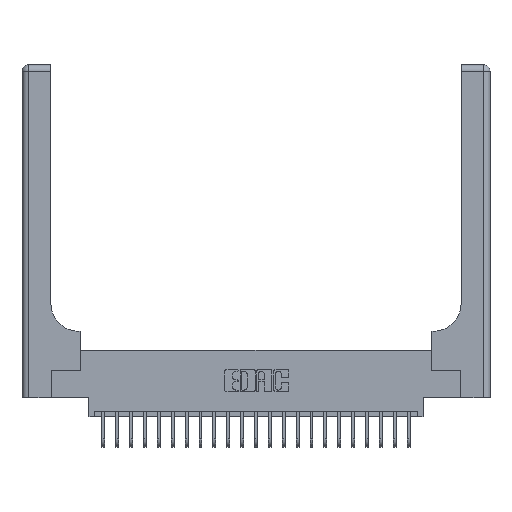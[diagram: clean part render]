
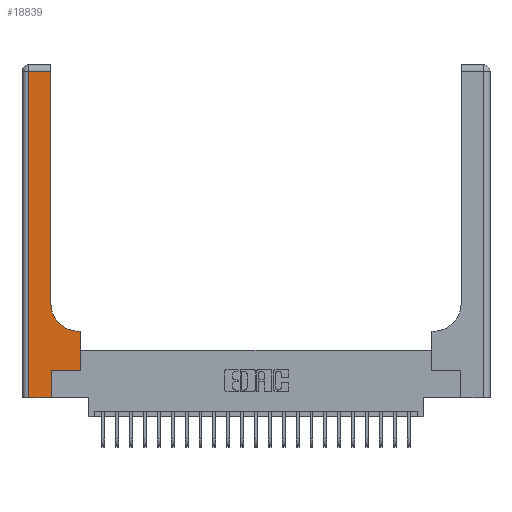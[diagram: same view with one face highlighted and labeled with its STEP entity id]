
A CAD part, top view. The second image highlights one B-rep face of the part: STEP entity #18839.
In plain terms, the highlighted planar face has unit normal (0, 0, 1).
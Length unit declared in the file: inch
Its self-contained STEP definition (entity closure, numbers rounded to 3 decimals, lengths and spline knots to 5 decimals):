
#45 = CARTESIAN_POINT ( 'NONE',  ( 0.51, 0.85, 0.37 ) ) ;
#279 = VERTEX_POINT ( 'NONE', #16182 ) ;
#375 = EDGE_CURVE ( 'NONE', #14481, #13839, #10200, .T. ) ;
#930 = LINE ( 'NONE', #8889, #1818 ) ;
#1572 = EDGE_CURVE ( 'NONE', #6969, #279, #13695, .T. ) ;
#1818 = VECTOR ( 'NONE', #12996, 39.37008 ) ;
#1852 = CARTESIAN_POINT ( 'NONE',  ( 0.06, 2.94, 0.37 ) ) ;
#2109 = ORIENTED_EDGE ( 'NONE', *, *, #14729, .T. ) ;
#2408 = DIRECTION ( 'NONE',  ( 1., 0., 0. ) ) ;
#2704 = VECTOR ( 'NONE', #4896, 39.37008 ) ;
#2709 = VERTEX_POINT ( 'NONE', #18155 ) ;
#3014 = CARTESIAN_POINT ( 'NONE',  ( 0.265, 0., 0.37 ) ) ;
#3131 = LINE ( 'NONE', #18366, #6955 ) ;
#3745 = EDGE_CURVE ( 'NONE', #18095, #14481, #22326, .T. ) ;
#4564 = ORIENTED_EDGE ( 'NONE', *, *, #11835, .T. ) ;
#4658 = LINE ( 'NONE', #8134, #10041 ) ;
#4896 = DIRECTION ( 'NONE',  ( 0., 1., 0. ) ) ;
#5174 = CARTESIAN_POINT ( 'NONE',  ( 0.26, 0.6, 0.37 ) ) ;
#5315 = AXIS2_PLACEMENT_3D ( 'NONE', #45, #13384, #21041 ) ;
#5909 = DIRECTION ( 'NONE',  ( 0., 0., -1. ) ) ;
#6440 = CARTESIAN_POINT ( 'NONE',  ( 0.528, 0.25, 0.37 ) ) ;
#6832 = DIRECTION ( 'NONE',  ( 1., 0., 0. ) ) ;
#6955 = VECTOR ( 'NONE', #16441, 39.37008 ) ;
#6969 = VERTEX_POINT ( 'NONE', #14373 ) ;
#7077 = DIRECTION ( 'NONE',  ( 0., 1., 0. ) ) ;
#7205 = VERTEX_POINT ( 'NONE', #1852 ) ;
#7296 = ORIENTED_EDGE ( 'NONE', *, *, #14107, .T. ) ;
#8134 = CARTESIAN_POINT ( 'NONE',  ( 0.265, 0.25, 0.37 ) ) ;
#8305 = ORIENTED_EDGE ( 'NONE', *, *, #375, .T. ) ;
#8889 = CARTESIAN_POINT ( 'NONE',  ( 0., 2.94, 0.37 ) ) ;
#9319 = EDGE_LOOP ( 'NONE', ( #18360, #21940, #4564, #7296, #2109, #10422, #13967, #8305, #23266 ) ) ;
#9759 = DIRECTION ( 'NONE',  ( -1., 0., 0. ) ) ;
#10041 = VECTOR ( 'NONE', #2408, 39.37008 ) ;
#10200 = LINE ( 'NONE', #5174, #20629 ) ;
#10422 = ORIENTED_EDGE ( 'NONE', *, *, #22167, .T. ) ;
#10571 = CARTESIAN_POINT ( 'NONE',  ( 0.06, 0., 0.37 ) ) ;
#10867 = EDGE_CURVE ( 'NONE', #13839, #6969, #19542, .T. ) ;
#11835 = EDGE_CURVE ( 'NONE', #7205, #21996, #3131, .T. ) ;
#11915 = VECTOR ( 'NONE', #7077, 39.37008 ) ;
#11971 = DIRECTION ( 'NONE',  ( 0., 1., 0. ) ) ;
#12144 = VECTOR ( 'NONE', #11971, 39.37008 ) ;
#12259 = VECTOR ( 'NONE', #6832, 39.37008 ) ;
#12650 = CARTESIAN_POINT ( 'NONE',  ( 0.528, 0.25, 0.37 ) ) ;
#12725 = CARTESIAN_POINT ( 'NONE',  ( 0.51, 0.6, 0.37 ) ) ;
#12996 = DIRECTION ( 'NONE',  ( -1., 0., 0. ) ) ;
#13286 = CARTESIAN_POINT ( 'NONE',  ( 0.265, 0., 0.37 ) ) ;
#13384 = DIRECTION ( 'NONE',  ( 0., 0., -1. ) ) ;
#13695 = LINE ( 'NONE', #22455, #11915 ) ;
#13818 = EDGE_CURVE ( 'NONE', #279, #7205, #930, .T. ) ;
#13839 = VERTEX_POINT ( 'NONE', #12725 ) ;
#13967 = ORIENTED_EDGE ( 'NONE', *, *, #3745, .T. ) ;
#14107 = EDGE_CURVE ( 'NONE', #21996, #15468, #17940, .T. ) ;
#14373 = CARTESIAN_POINT ( 'NONE',  ( 0.26, 0.85, 0.37 ) ) ;
#14481 = VERTEX_POINT ( 'NONE', #17111 ) ;
#14729 = EDGE_CURVE ( 'NONE', #15468, #2709, #14930, .T. ) ;
#14930 = LINE ( 'NONE', #3014, #2704 ) ;
#15468 = VERTEX_POINT ( 'NONE', #13286 ) ;
#15819 = FACE_OUTER_BOUND ( 'NONE', #9319, .T. ) ;
#16182 = CARTESIAN_POINT ( 'NONE',  ( 0.26, 2.94, 0.37 ) ) ;
#16441 = DIRECTION ( 'NONE',  ( 0., -1., 0. ) ) ;
#17111 = CARTESIAN_POINT ( 'NONE',  ( 0.528, 0.6, 0.37 ) ) ;
#17300 = PLANE ( 'NONE',  #23432 ) ;
#17380 = CARTESIAN_POINT ( 'NONE',  ( 0., 3., 0.37 ) ) ;
#17940 = LINE ( 'NONE', #23045, #12259 ) ;
#18095 = VERTEX_POINT ( 'NONE', #12650 ) ;
#18155 = CARTESIAN_POINT ( 'NONE',  ( 0.265, 0.25, 0.37 ) ) ;
#18360 = ORIENTED_EDGE ( 'NONE', *, *, #1572, .T. ) ;
#18366 = CARTESIAN_POINT ( 'NONE',  ( 0.06, 3., 0.37 ) ) ;
#18497 = DIRECTION ( 'NONE',  ( -1., 0., 0. ) ) ;
#18839 = ADVANCED_FACE ( 'NONE', ( #15819 ), #17300, .F. ) ;
#19542 = CIRCLE ( 'NONE', #5315, 0.25 ) ;
#20629 = VECTOR ( 'NONE', #18497, 39.37008 ) ;
#21041 = DIRECTION ( 'NONE',  ( 1., 0., 0. ) ) ;
#21940 = ORIENTED_EDGE ( 'NONE', *, *, #13818, .T. ) ;
#21996 = VERTEX_POINT ( 'NONE', #10571 ) ;
#22167 = EDGE_CURVE ( 'NONE', #2709, #18095, #4658, .T. ) ;
#22326 = LINE ( 'NONE', #6440, #12144 ) ;
#22455 = CARTESIAN_POINT ( 'NONE',  ( 0.26, 3., 0.37 ) ) ;
#23045 = CARTESIAN_POINT ( 'NONE',  ( 0., 0., 0.37 ) ) ;
#23266 = ORIENTED_EDGE ( 'NONE', *, *, #10867, .T. ) ;
#23432 = AXIS2_PLACEMENT_3D ( 'NONE', #17380, #5909, #9759 ) ;
